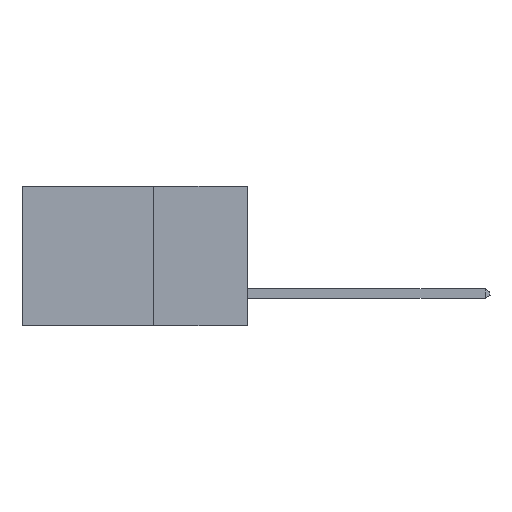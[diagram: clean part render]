
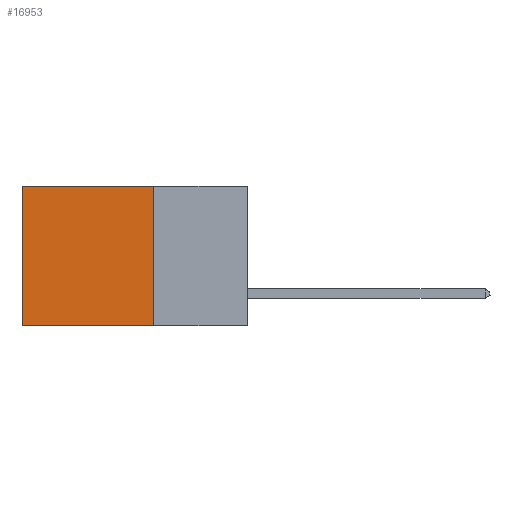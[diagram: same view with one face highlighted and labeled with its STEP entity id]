
A CAD part, left-side view. The second image highlights one B-rep face of the part: STEP entity #16953.
In plain terms, the highlighted planar face has unit normal (-1, 0, 0).
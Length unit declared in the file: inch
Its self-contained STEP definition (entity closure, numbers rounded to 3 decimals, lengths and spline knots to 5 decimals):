
#1792 = ORIENTED_EDGE ( 'NONE', *, *, #5345, .F. ) ;
#3242 = CARTESIAN_POINT ( 'NONE',  ( 0.298, 0.25, 0. ) ) ;
#4218 = ORIENTED_EDGE ( 'NONE', *, *, #22734, .T. ) ;
#4363 = AXIS2_PLACEMENT_3D ( 'NONE', #23259, #6156, #8309 ) ;
#4904 = EDGE_CURVE ( 'NONE', #23735, #21683, #17786, .T. ) ;
#5345 = EDGE_CURVE ( 'NONE', #21683, #24181, #19852, .T. ) ;
#5615 = CARTESIAN_POINT ( 'NONE',  ( 0.298, 0.25, 0. ) ) ;
#5649 = CARTESIAN_POINT ( 'NONE',  ( 0.298, 0.25, -0.37 ) ) ;
#6156 = DIRECTION ( 'NONE',  ( 1., 0., 0. ) ) ;
#6233 = EDGE_LOOP ( 'NONE', ( #4218, #1792, #15989, #15157 ) ) ;
#6973 = DIRECTION ( 'NONE',  ( 0., 0., -1. ) ) ;
#7117 = CARTESIAN_POINT ( 'NONE',  ( 0.298, 0.25, 0. ) ) ;
#7289 = FACE_OUTER_BOUND ( 'NONE', #6233, .T. ) ;
#7823 = VERTEX_POINT ( 'NONE', #17409 ) ;
#8191 = CARTESIAN_POINT ( 'NONE',  ( 0.298, 0.25, -0.37 ) ) ;
#8309 = DIRECTION ( 'NONE',  ( 0., 0., -1. ) ) ;
#10630 = VECTOR ( 'NONE', #13113, 39.37008 ) ;
#11633 = DIRECTION ( 'NONE',  ( 0., 1., 0. ) ) ;
#13113 = DIRECTION ( 'NONE',  ( 0., 1., 0. ) ) ;
#15157 = ORIENTED_EDGE ( 'NONE', *, *, #19892, .T. ) ;
#15655 = LINE ( 'NONE', #5615, #10630 ) ;
#15989 = ORIENTED_EDGE ( 'NONE', *, *, #4904, .F. ) ;
#16920 = VECTOR ( 'NONE', #11633, 39.37008 ) ;
#16953 = ADVANCED_FACE ( 'NONE', ( #7289 ), #19620, .F. ) ;
#17409 = CARTESIAN_POINT ( 'NONE',  ( 0.298, 0.6, 0. ) ) ;
#17786 = LINE ( 'NONE', #3242, #23712 ) ;
#18353 = DIRECTION ( 'NONE',  ( 0., 0., -1. ) ) ;
#19620 = PLANE ( 'NONE',  #4363 ) ;
#19852 = LINE ( 'NONE', #5649, #16920 ) ;
#19892 = EDGE_CURVE ( 'NONE', #23735, #7823, #15655, .T. ) ;
#21132 = VECTOR ( 'NONE', #6973, 39.37008 ) ;
#21683 = VERTEX_POINT ( 'NONE', #8191 ) ;
#21916 = CARTESIAN_POINT ( 'NONE',  ( 0.298, 0.6, 0. ) ) ;
#22013 = LINE ( 'NONE', #21916, #21132 ) ;
#22734 = EDGE_CURVE ( 'NONE', #7823, #24181, #22013, .T. ) ;
#23259 = CARTESIAN_POINT ( 'NONE',  ( 0.298, 0.25, 0. ) ) ;
#23712 = VECTOR ( 'NONE', #18353, 39.37008 ) ;
#23735 = VERTEX_POINT ( 'NONE', #7117 ) ;
#24181 = VERTEX_POINT ( 'NONE', #24488 ) ;
#24488 = CARTESIAN_POINT ( 'NONE',  ( 0.298, 0.6, -0.37 ) ) ;
